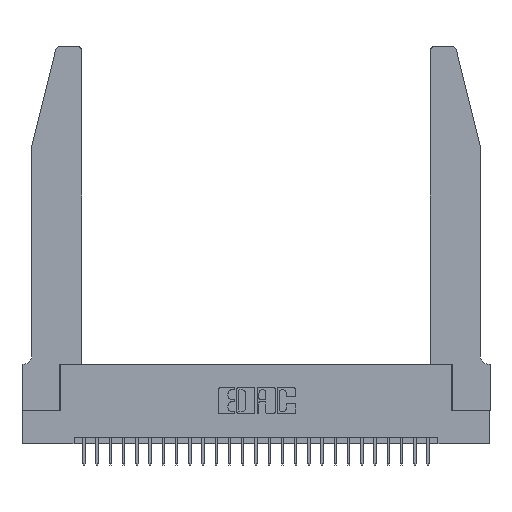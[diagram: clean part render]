
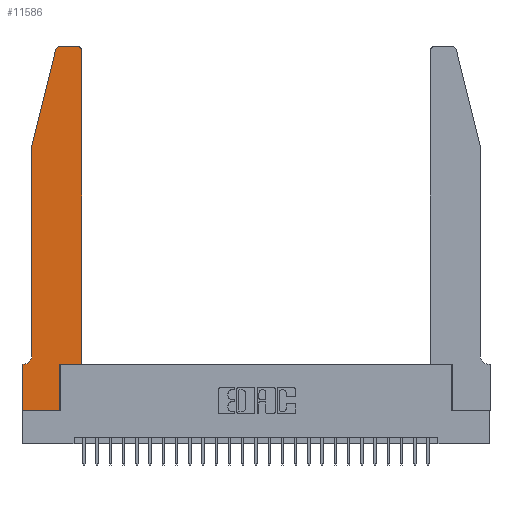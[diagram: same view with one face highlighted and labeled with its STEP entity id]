
A CAD part, top view. The second image highlights one B-rep face of the part: STEP entity #11586.
In plain terms, the highlighted planar face has unit normal (0, 0, 1).
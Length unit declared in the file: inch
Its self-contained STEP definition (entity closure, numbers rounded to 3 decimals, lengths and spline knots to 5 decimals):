
#292 = VECTOR ( 'NONE', #22130, 39.37008 ) ;
#563 = LINE ( 'NONE', #14248, #23608 ) ;
#832 = ORIENTED_EDGE ( 'NONE', *, *, #5135, .T. ) ;
#1534 = DIRECTION ( 'NONE',  ( 0., -1., 0. ) ) ;
#2441 = VECTOR ( 'NONE', #1534, 39.37008 ) ;
#2628 = CARTESIAN_POINT ( 'NONE',  ( 0.0755, 0.42, 0.37 ) ) ;
#2802 = ORIENTED_EDGE ( 'NONE', *, *, #5649, .T. ) ;
#2897 = FACE_OUTER_BOUND ( 'NONE', #5567, .T. ) ;
#3139 = VERTEX_POINT ( 'NONE', #20637 ) ;
#3219 = LINE ( 'NONE', #4566, #9001 ) ;
#3422 = DIRECTION ( 'NONE',  ( -1., 0., 0. ) ) ;
#3900 = CARTESIAN_POINT ( 'NONE',  ( 0.4205, 2.72, 0.37 ) ) ;
#4062 = EDGE_CURVE ( 'NONE', #3139, #26652, #3219, .T. ) ;
#4179 = VERTEX_POINT ( 'NONE', #20042 ) ;
#4261 = ORIENTED_EDGE ( 'NONE', *, *, #9146, .T. ) ;
#4566 = CARTESIAN_POINT ( 'NONE',  ( 0., 0., 0.37 ) ) ;
#4657 = VERTEX_POINT ( 'NONE', #26852 ) ;
#4892 = DIRECTION ( 'NONE',  ( 0., 1., 0. ) ) ;
#5135 = EDGE_CURVE ( 'NONE', #4657, #17255, #12363, .T. ) ;
#5567 = EDGE_LOOP ( 'NONE', ( #4261, #13084, #832, #26958, #6531, #27696, #27727, #7603, #16043, #2802, #16398, #12026 ) ) ;
#5649 = EDGE_CURVE ( 'NONE', #4179, #9964, #11677, .T. ) ;
#6088 = DIRECTION ( 'NONE',  ( 1., 0., 0. ) ) ;
#6420 = EDGE_CURVE ( 'NONE', #26652, #4179, #26368, .T. ) ;
#6476 = EDGE_CURVE ( 'NONE', #23999, #4657, #8576, .T. ) ;
#6531 = ORIENTED_EDGE ( 'NONE', *, *, #13620, .T. ) ;
#6541 = EDGE_CURVE ( 'NONE', #13935, #9674, #14335, .T. ) ;
#6689 = VECTOR ( 'NONE', #12641, 39.37008 ) ;
#6804 = AXIS2_PLACEMENT_3D ( 'NONE', #12334, #27318, #14513 ) ;
#6892 = LINE ( 'NONE', #11342, #292 ) ;
#7603 = ORIENTED_EDGE ( 'NONE', *, *, #4062, .T. ) ;
#7616 = LINE ( 'NONE', #16803, #2441 ) ;
#8576 = CIRCLE ( 'NONE', #6804, 0.03 ) ;
#9001 = VECTOR ( 'NONE', #19674, 39.37008 ) ;
#9038 = CARTESIAN_POINT ( 'NONE',  ( 0.4505, 2.72, 0.37 ) ) ;
#9146 = EDGE_CURVE ( 'NONE', #9674, #23999, #563, .T. ) ;
#9418 = AXIS2_PLACEMENT_3D ( 'NONE', #25867, #12958, #17385 ) ;
#9674 = VERTEX_POINT ( 'NONE', #22716 ) ;
#9964 = VERTEX_POINT ( 'NONE', #19651 ) ;
#11342 = CARTESIAN_POINT ( 'NONE',  ( 0., 0., 0.37 ) ) ;
#11497 = CARTESIAN_POINT ( 'NONE',  ( 0., 0.35, 0.37 ) ) ;
#11579 = CARTESIAN_POINT ( 'NONE',  ( 0.0755, 2., 0.37 ) ) ;
#11586 = ADVANCED_FACE ( 'NONE', ( #2897 ), #15228, .T. ) ;
#11677 = LINE ( 'NONE', #25953, #23711 ) ;
#12026 = ORIENTED_EDGE ( 'NONE', *, *, #6541, .T. ) ;
#12168 = LINE ( 'NONE', #15668, #22887 ) ;
#12184 = CARTESIAN_POINT ( 'NONE',  ( 0.0055, 0.42, 0.37 ) ) ;
#12334 = CARTESIAN_POINT ( 'NONE',  ( 0.284, 2.72, 0.37 ) ) ;
#12363 = LINE ( 'NONE', #11579, #17419 ) ;
#12590 = AXIS2_PLACEMENT_3D ( 'NONE', #3900, #19021, #6088 ) ;
#12641 = DIRECTION ( 'NONE',  ( -1., 0., 0. ) ) ;
#12958 = DIRECTION ( 'NONE',  ( 0., 0., 1. ) ) ;
#13084 = ORIENTED_EDGE ( 'NONE', *, *, #6476, .T. ) ;
#13120 = LINE ( 'NONE', #25928, #6689 ) ;
#13620 = EDGE_CURVE ( 'NONE', #27295, #17634, #19154, .T. ) ;
#13935 = VERTEX_POINT ( 'NONE', #9038 ) ;
#14026 = VERTEX_POINT ( 'NONE', #11497 ) ;
#14248 = CARTESIAN_POINT ( 'NONE',  ( 0.2605, 2.75, 0.37 ) ) ;
#14251 = DIRECTION ( 'NONE',  ( 0., 1., 0. ) ) ;
#14335 = CIRCLE ( 'NONE', #12590, 0.03 ) ;
#14360 = DIRECTION ( 'NONE',  ( -1., 0., 0. ) ) ;
#14513 = DIRECTION ( 'NONE',  ( 1., 0., 0. ) ) ;
#15228 = PLANE ( 'NONE',  #9418 ) ;
#15501 = CARTESIAN_POINT ( 'NONE',  ( 0.2865, 0., 0.37 ) ) ;
#15668 = CARTESIAN_POINT ( 'NONE',  ( 0.4505, 0.35, 0.37 ) ) ;
#16043 = ORIENTED_EDGE ( 'NONE', *, *, #6420, .T. ) ;
#16398 = ORIENTED_EDGE ( 'NONE', *, *, #21079, .T. ) ;
#16405 = CARTESIAN_POINT ( 'NONE',  ( 0.2865, 0.35, 0.37 ) ) ;
#16803 = CARTESIAN_POINT ( 'NONE',  ( 0.0755, 2., 0.37 ) ) ;
#17255 = VERTEX_POINT ( 'NONE', #21874 ) ;
#17385 = DIRECTION ( 'NONE',  ( 1., 0., 0. ) ) ;
#17419 = VECTOR ( 'NONE', #26463, 39.37008 ) ;
#17634 = VERTEX_POINT ( 'NONE', #20921 ) ;
#19021 = DIRECTION ( 'NONE',  ( 0., 0., 1. ) ) ;
#19154 = CIRCLE ( 'NONE', #19772, 0.07 ) ;
#19651 = CARTESIAN_POINT ( 'NONE',  ( 0.4505, 0.35, 0.37 ) ) ;
#19674 = DIRECTION ( 'NONE',  ( 1., 0., 0. ) ) ;
#19772 = AXIS2_PLACEMENT_3D ( 'NONE', #12184, #27166, #14360 ) ;
#20042 = CARTESIAN_POINT ( 'NONE',  ( 0.2865, 0.35, 0.37 ) ) ;
#20149 = CARTESIAN_POINT ( 'NONE',  ( 0.284, 2.75, 0.37 ) ) ;
#20637 = CARTESIAN_POINT ( 'NONE',  ( 0., 0., 0.37 ) ) ;
#20691 = VECTOR ( 'NONE', #14251, 39.37008 ) ;
#20921 = CARTESIAN_POINT ( 'NONE',  ( 0.0055, 0.35, 0.37 ) ) ;
#21079 = EDGE_CURVE ( 'NONE', #9964, #13935, #12168, .T. ) ;
#21768 = DIRECTION ( 'NONE',  ( 1., 0., 0. ) ) ;
#21874 = CARTESIAN_POINT ( 'NONE',  ( 0.0755, 2., 0.37 ) ) ;
#22130 = DIRECTION ( 'NONE',  ( 0., -1., 0. ) ) ;
#22716 = CARTESIAN_POINT ( 'NONE',  ( 0.4205, 2.75, 0.37 ) ) ;
#22887 = VECTOR ( 'NONE', #4892, 39.37008 ) ;
#23589 = EDGE_CURVE ( 'NONE', #17255, #27295, #7616, .T. ) ;
#23608 = VECTOR ( 'NONE', #3422, 39.37008 ) ;
#23711 = VECTOR ( 'NONE', #21768, 39.37008 ) ;
#23999 = VERTEX_POINT ( 'NONE', #20149 ) ;
#24812 = EDGE_CURVE ( 'NONE', #14026, #3139, #6892, .T. ) ;
#25867 = CARTESIAN_POINT ( 'NONE',  ( 0., 0.35, 0.37 ) ) ;
#25928 = CARTESIAN_POINT ( 'NONE',  ( 0.0755, 0.35, 0.37 ) ) ;
#25953 = CARTESIAN_POINT ( 'NONE',  ( 0.4505, 0.35, 0.37 ) ) ;
#26368 = LINE ( 'NONE', #16405, #20691 ) ;
#26463 = DIRECTION ( 'NONE',  ( -0.239, -0.971, 0. ) ) ;
#26652 = VERTEX_POINT ( 'NONE', #15501 ) ;
#26852 = CARTESIAN_POINT ( 'NONE',  ( 0.25487, 2.72718, 0.37 ) ) ;
#26958 = ORIENTED_EDGE ( 'NONE', *, *, #23589, .T. ) ;
#27166 = DIRECTION ( 'NONE',  ( 0., 0., -1. ) ) ;
#27295 = VERTEX_POINT ( 'NONE', #2628 ) ;
#27318 = DIRECTION ( 'NONE',  ( 0., 0., 1. ) ) ;
#27592 = EDGE_CURVE ( 'NONE', #17634, #14026, #13120, .T. ) ;
#27696 = ORIENTED_EDGE ( 'NONE', *, *, #27592, .T. ) ;
#27727 = ORIENTED_EDGE ( 'NONE', *, *, #24812, .T. ) ;
